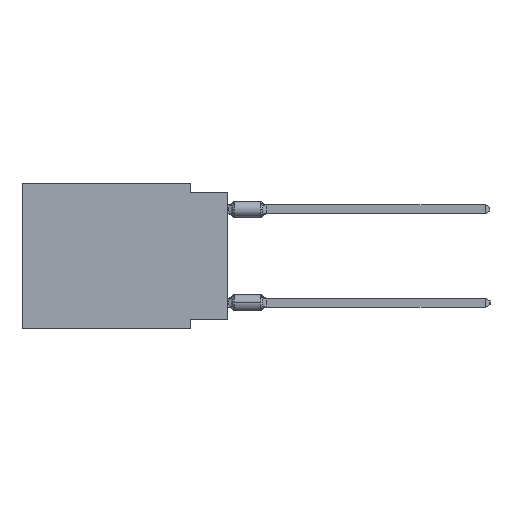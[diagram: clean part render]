
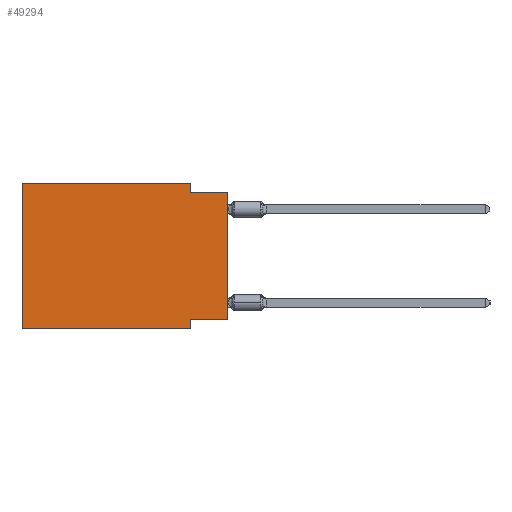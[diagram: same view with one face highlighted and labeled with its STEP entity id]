
A CAD part, left-side view. The second image highlights one B-rep face of the part: STEP entity #49294.
In plain terms, the highlighted planar face has unit normal (-1, 0, 0).
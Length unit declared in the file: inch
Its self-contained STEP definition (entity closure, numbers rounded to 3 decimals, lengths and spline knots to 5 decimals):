
#178 = CARTESIAN_POINT ( 'NONE',  ( 0., 0.55, 0. ) ) ;
#1051 = ORIENTED_EDGE ( 'NONE', *, *, #19403, .F. ) ;
#2272 = CARTESIAN_POINT ( 'NONE',  ( 0., 0.1, -0.365 ) ) ;
#3810 = CARTESIAN_POINT ( 'NONE',  ( 0., 0.55, -0.39 ) ) ;
#4420 = LINE ( 'NONE', #24480, #28915 ) ;
#5304 = CARTESIAN_POINT ( 'NONE',  ( 0., 0.55, 0. ) ) ;
#6162 = ORIENTED_EDGE ( 'NONE', *, *, #43710, .F. ) ;
#8740 = DIRECTION ( 'NONE',  ( 0., -1., 0. ) ) ;
#9103 = EDGE_CURVE ( 'NONE', #18591, #17705, #47372, .T. ) ;
#10087 = DIRECTION ( 'NONE',  ( 1., 0., 0. ) ) ;
#10355 = VECTOR ( 'NONE', #55988, 39.37008 ) ;
#10537 = CARTESIAN_POINT ( 'NONE',  ( 0., 0.1, -0.025 ) ) ;
#17086 = EDGE_CURVE ( 'NONE', #58066, #57740, #21283, .T. ) ;
#17667 = DIRECTION ( 'NONE',  ( 0., 0., 1. ) ) ;
#17705 = VERTEX_POINT ( 'NONE', #178 ) ;
#18359 = CARTESIAN_POINT ( 'NONE',  ( 0., 0.1, -0.39 ) ) ;
#18591 = VERTEX_POINT ( 'NONE', #3810 ) ;
#19178 = FACE_OUTER_BOUND ( 'NONE', #24619, .T. ) ;
#19183 = VERTEX_POINT ( 'NONE', #10537 ) ;
#19403 = EDGE_CURVE ( 'NONE', #49068, #19183, #61620, .T. ) ;
#20270 = ORIENTED_EDGE ( 'NONE', *, *, #59625, .F. ) ;
#21283 = LINE ( 'NONE', #40432, #37231 ) ;
#22516 = ORIENTED_EDGE ( 'NONE', *, *, #51360, .T. ) ;
#23316 = AXIS2_PLACEMENT_3D ( 'NONE', #53084, #10087, #40161 ) ;
#23544 = DIRECTION ( 'NONE',  ( 0., -1., 0. ) ) ;
#24124 = DIRECTION ( 'NONE',  ( 0., 0., 1. ) ) ;
#24480 = CARTESIAN_POINT ( 'NONE',  ( 0., 0., -0.025 ) ) ;
#24619 = EDGE_LOOP ( 'NONE', ( #22516, #6162, #1051, #59307, #60476, #31655, #20270, #29409 ) ) ;
#24639 = CARTESIAN_POINT ( 'NONE',  ( 0., 0., -0.025 ) ) ;
#27441 = VECTOR ( 'NONE', #56925, 39.37008 ) ;
#27872 = LINE ( 'NONE', #51751, #50232 ) ;
#28915 = VECTOR ( 'NONE', #23544, 39.37008 ) ;
#29409 = ORIENTED_EDGE ( 'NONE', *, *, #17086, .F. ) ;
#31655 = ORIENTED_EDGE ( 'NONE', *, *, #49174, .T. ) ;
#37231 = VECTOR ( 'NONE', #52829, 39.37008 ) ;
#37761 = CARTESIAN_POINT ( 'NONE',  ( 0., 0.1, 0. ) ) ;
#38310 = CARTESIAN_POINT ( 'NONE',  ( 0., 0.55, -0.39 ) ) ;
#38417 = VECTOR ( 'NONE', #17667, 39.37008 ) ;
#40118 = LINE ( 'NONE', #41280, #40961 ) ;
#40161 = DIRECTION ( 'NONE',  ( 0., 0., -1. ) ) ;
#40432 = CARTESIAN_POINT ( 'NONE',  ( 0., 0., -0.365 ) ) ;
#40961 = VECTOR ( 'NONE', #58982, 39.37008 ) ;
#41280 = CARTESIAN_POINT ( 'NONE',  ( 0., 0.1, -0.39 ) ) ;
#43292 = CARTESIAN_POINT ( 'NONE',  ( 0., 0., 0. ) ) ;
#43710 = EDGE_CURVE ( 'NONE', #19183, #44632, #4420, .T. ) ;
#44632 = VERTEX_POINT ( 'NONE', #24639 ) ;
#47213 = EDGE_CURVE ( 'NONE', #17705, #49068, #27872, .T. ) ;
#47372 = LINE ( 'NONE', #5304, #49776 ) ;
#48054 = PLANE ( 'NONE',  #23316 ) ;
#49068 = VERTEX_POINT ( 'NONE', #59763 ) ;
#49174 = EDGE_CURVE ( 'NONE', #18591, #50961, #56298, .T. ) ;
#49294 = ADVANCED_FACE ( 'NONE', ( #19178 ), #48054, .F. ) ;
#49776 = VECTOR ( 'NONE', #24124, 39.37008 ) ;
#50232 = VECTOR ( 'NONE', #8740, 39.37008 ) ;
#50961 = VERTEX_POINT ( 'NONE', #18359 ) ;
#51360 = EDGE_CURVE ( 'NONE', #58066, #44632, #53050, .T. ) ;
#51751 = CARTESIAN_POINT ( 'NONE',  ( 0., 0.55, 0. ) ) ;
#52829 = DIRECTION ( 'NONE',  ( 0., 1., 0. ) ) ;
#53050 = LINE ( 'NONE', #43292, #38417 ) ;
#53084 = CARTESIAN_POINT ( 'NONE',  ( 0., 0.55, 0. ) ) ;
#53382 = CARTESIAN_POINT ( 'NONE',  ( 0., 0., -0.365 ) ) ;
#55988 = DIRECTION ( 'NONE',  ( 0., -1., 0. ) ) ;
#56298 = LINE ( 'NONE', #38310, #10355 ) ;
#56925 = DIRECTION ( 'NONE',  ( 0., 0., -1. ) ) ;
#57740 = VERTEX_POINT ( 'NONE', #2272 ) ;
#58066 = VERTEX_POINT ( 'NONE', #53382 ) ;
#58982 = DIRECTION ( 'NONE',  ( 0., 0., -1. ) ) ;
#59307 = ORIENTED_EDGE ( 'NONE', *, *, #47213, .F. ) ;
#59625 = EDGE_CURVE ( 'NONE', #57740, #50961, #40118, .T. ) ;
#59763 = CARTESIAN_POINT ( 'NONE',  ( 0., 0.1, 0. ) ) ;
#60476 = ORIENTED_EDGE ( 'NONE', *, *, #9103, .F. ) ;
#61620 = LINE ( 'NONE', #37761, #27441 ) ;
